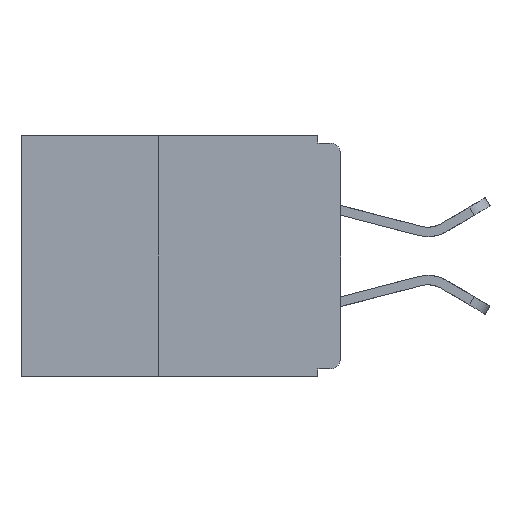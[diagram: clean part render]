
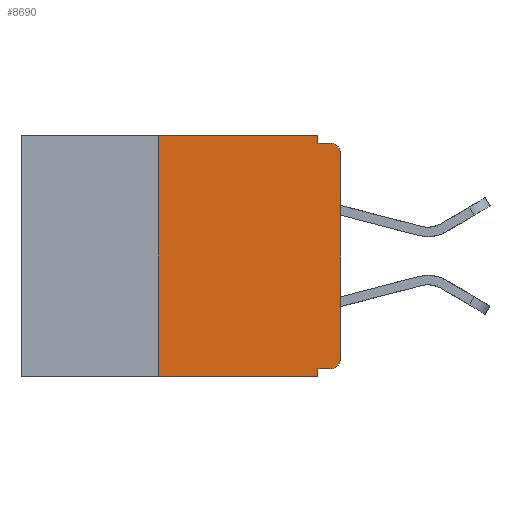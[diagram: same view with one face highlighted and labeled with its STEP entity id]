
A CAD part, left-side view. The second image highlights one B-rep face of the part: STEP entity #8690.
In plain terms, the highlighted planar face has unit normal (-1, 0, 0).
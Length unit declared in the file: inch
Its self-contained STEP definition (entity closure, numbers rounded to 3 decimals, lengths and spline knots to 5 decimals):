
#82 = CARTESIAN_POINT ( 'NONE',  ( 0., 0.031, -0.01 ) ) ;
#1064 = DIRECTION ( 'NONE',  ( 0., 1., 0. ) ) ;
#1430 = CARTESIAN_POINT ( 'NONE',  ( 0., 0.031, 0. ) ) ;
#1567 = FACE_OUTER_BOUND ( 'NONE', #8212, .T. ) ;
#1572 = CARTESIAN_POINT ( 'NONE',  ( 0., 0.031, 0. ) ) ;
#1587 = AXIS2_PLACEMENT_3D ( 'NONE', #13518, #29064, #15803 ) ;
#2061 = VERTEX_POINT ( 'NONE', #1572 ) ;
#2779 = CARTESIAN_POINT ( 'NONE',  ( 0., 0.031, -0.33 ) ) ;
#3745 = AXIS2_PLACEMENT_3D ( 'NONE', #24557, #28981, #15728 ) ;
#5305 = EDGE_CURVE ( 'NONE', #2061, #27453, #8664, .T. ) ;
#5601 = DIRECTION ( 'NONE',  ( 0., 0., 1. ) ) ;
#5739 = CIRCLE ( 'NONE', #1587, 0.015 ) ;
#6188 = CARTESIAN_POINT ( 'NONE',  ( 0., 0., -0.025 ) ) ;
#6483 = ORIENTED_EDGE ( 'NONE', *, *, #23333, .T. ) ;
#6785 = EDGE_CURVE ( 'NONE', #10319, #24850, #5739, .T. ) ;
#7664 = DIRECTION ( 'NONE',  ( -1., 0., 0. ) ) ;
#8212 = EDGE_LOOP ( 'NONE', ( #6483, #10431, #16267, #20041, #20388, #24068, #11958, #12804, #23251, #25481 ) ) ;
#8336 = VECTOR ( 'NONE', #15458, 39.37008 ) ;
#8390 = EDGE_CURVE ( 'NONE', #24355, #8998, #21296, .T. ) ;
#8664 = LINE ( 'NONE', #1430, #10053 ) ;
#8690 = ADVANCED_FACE ( 'NONE', ( #1567 ), #20117, .F. ) ;
#8726 = LINE ( 'NONE', #15012, #13998 ) ;
#8998 = VERTEX_POINT ( 'NONE', #19133 ) ;
#9303 = AXIS2_PLACEMENT_3D ( 'NONE', #21073, #7664, #23284 ) ;
#9437 = CARTESIAN_POINT ( 'NONE',  ( 0., 0.25, -0.33 ) ) ;
#9613 = DIRECTION ( 'NONE',  ( 0., 0., -1. ) ) ;
#9759 = VERTEX_POINT ( 'NONE', #15082 ) ;
#10024 = CARTESIAN_POINT ( 'NONE',  ( 0., 0.25, -0.33 ) ) ;
#10053 = VECTOR ( 'NONE', #19506, 39.37008 ) ;
#10319 = VERTEX_POINT ( 'NONE', #6188 ) ;
#10431 = ORIENTED_EDGE ( 'NONE', *, *, #6785, .T. ) ;
#10886 = VERTEX_POINT ( 'NONE', #23376 ) ;
#10915 = VECTOR ( 'NONE', #15702, 39.37008 ) ;
#10929 = CARTESIAN_POINT ( 'NONE',  ( 0., 0.437, -0.33 ) ) ;
#11270 = CIRCLE ( 'NONE', #9303, 0.015 ) ;
#11567 = CARTESIAN_POINT ( 'NONE',  ( 0., 0., -0.01 ) ) ;
#11958 = ORIENTED_EDGE ( 'NONE', *, *, #18603, .T. ) ;
#12634 = LINE ( 'NONE', #11567, #23800 ) ;
#12804 = ORIENTED_EDGE ( 'NONE', *, *, #19736, .F. ) ;
#13421 = CARTESIAN_POINT ( 'NONE',  ( 0., 0.437, 0. ) ) ;
#13518 = CARTESIAN_POINT ( 'NONE',  ( 0., 0.015, -0.025 ) ) ;
#13821 = DIRECTION ( 'NONE',  ( 0., -1., 0. ) ) ;
#13998 = VECTOR ( 'NONE', #23939, 39.37008 ) ;
#14319 = LINE ( 'NONE', #10929, #8336 ) ;
#15012 = CARTESIAN_POINT ( 'NONE',  ( 0., 0., 0. ) ) ;
#15054 = VECTOR ( 'NONE', #1064, 39.37008 ) ;
#15082 = CARTESIAN_POINT ( 'NONE',  ( 0., 0.031, -0.33 ) ) ;
#15458 = DIRECTION ( 'NONE',  ( 0., -1., 0. ) ) ;
#15702 = DIRECTION ( 'NONE',  ( 0., -1., 0. ) ) ;
#15728 = DIRECTION ( 'NONE',  ( 0., 0., -1. ) ) ;
#15756 = LINE ( 'NONE', #27962, #15054 ) ;
#15803 = DIRECTION ( 'NONE',  ( 0., 0., -1. ) ) ;
#15839 = EDGE_CURVE ( 'NONE', #8998, #2061, #28682, .T. ) ;
#16267 = ORIENTED_EDGE ( 'NONE', *, *, #22094, .F. ) ;
#17763 = VECTOR ( 'NONE', #9613, 39.37008 ) ;
#18484 = LINE ( 'NONE', #2779, #17763 ) ;
#18603 = EDGE_CURVE ( 'NONE', #24355, #9759, #14319, .T. ) ;
#18763 = VERTEX_POINT ( 'NONE', #27150 ) ;
#19133 = CARTESIAN_POINT ( 'NONE',  ( 0., 0.25, 0. ) ) ;
#19506 = DIRECTION ( 'NONE',  ( 0., 0., -1. ) ) ;
#19736 = EDGE_CURVE ( 'NONE', #18763, #9759, #18484, .T. ) ;
#20041 = ORIENTED_EDGE ( 'NONE', *, *, #5305, .F. ) ;
#20117 = PLANE ( 'NONE',  #3745 ) ;
#20388 = ORIENTED_EDGE ( 'NONE', *, *, #15839, .F. ) ;
#21073 = CARTESIAN_POINT ( 'NONE',  ( 0., 0.015, -0.305 ) ) ;
#21092 = EDGE_CURVE ( 'NONE', #21183, #10886, #11270, .T. ) ;
#21183 = VERTEX_POINT ( 'NONE', #23569 ) ;
#21296 = LINE ( 'NONE', #10024, #26548 ) ;
#22094 = EDGE_CURVE ( 'NONE', #27453, #24850, #12634, .T. ) ;
#23251 = ORIENTED_EDGE ( 'NONE', *, *, #26580, .F. ) ;
#23284 = DIRECTION ( 'NONE',  ( 0., 0., -1. ) ) ;
#23333 = EDGE_CURVE ( 'NONE', #10886, #10319, #8726, .T. ) ;
#23376 = CARTESIAN_POINT ( 'NONE',  ( 0., 0., -0.305 ) ) ;
#23569 = CARTESIAN_POINT ( 'NONE',  ( 0., 0.015, -0.32 ) ) ;
#23800 = VECTOR ( 'NONE', #13821, 39.37008 ) ;
#23939 = DIRECTION ( 'NONE',  ( 0., 0., 1. ) ) ;
#24068 = ORIENTED_EDGE ( 'NONE', *, *, #8390, .F. ) ;
#24355 = VERTEX_POINT ( 'NONE', #9437 ) ;
#24557 = CARTESIAN_POINT ( 'NONE',  ( 0., 0.437, 0. ) ) ;
#24850 = VERTEX_POINT ( 'NONE', #26715 ) ;
#25481 = ORIENTED_EDGE ( 'NONE', *, *, #21092, .T. ) ;
#26548 = VECTOR ( 'NONE', #5601, 39.37008 ) ;
#26580 = EDGE_CURVE ( 'NONE', #21183, #18763, #15756, .T. ) ;
#26715 = CARTESIAN_POINT ( 'NONE',  ( 0., 0.015, -0.01 ) ) ;
#27150 = CARTESIAN_POINT ( 'NONE',  ( 0., 0.031, -0.32 ) ) ;
#27453 = VERTEX_POINT ( 'NONE', #82 ) ;
#27962 = CARTESIAN_POINT ( 'NONE',  ( 0., 0., -0.32 ) ) ;
#28682 = LINE ( 'NONE', #13421, #10915 ) ;
#28981 = DIRECTION ( 'NONE',  ( 1., 0., 0. ) ) ;
#29064 = DIRECTION ( 'NONE',  ( -1., 0., 0. ) ) ;
